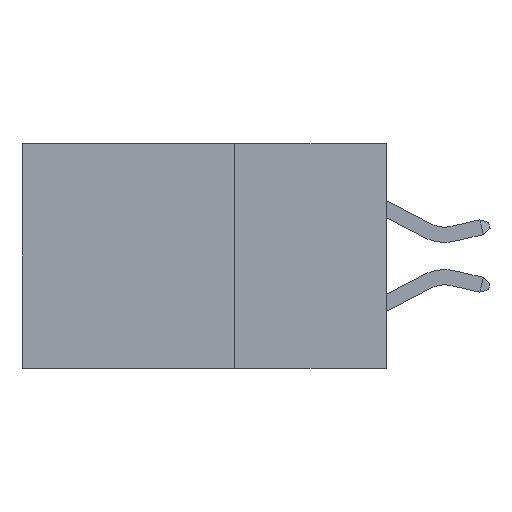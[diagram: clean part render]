
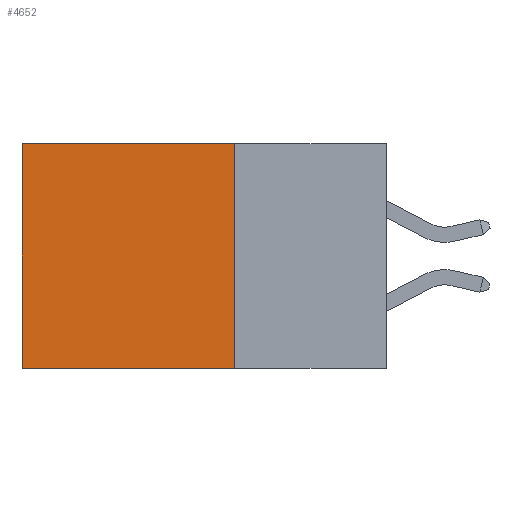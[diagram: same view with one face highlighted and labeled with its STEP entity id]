
A CAD part, left-side view. The second image highlights one B-rep face of the part: STEP entity #4652.
In plain terms, the highlighted planar face has unit normal (-1, 0, 0).
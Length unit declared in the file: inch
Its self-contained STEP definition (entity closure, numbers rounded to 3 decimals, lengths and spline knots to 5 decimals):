
#486 = VERTEX_POINT ( 'NONE', #7137 ) ;
#935 = DIRECTION ( 'NONE',  ( 0., 0., -1. ) ) ;
#1513 = EDGE_LOOP ( 'NONE', ( #7203, #8197, #4393, #14992 ) ) ;
#1805 = VERTEX_POINT ( 'NONE', #5164 ) ;
#1903 = VECTOR ( 'NONE', #11298, 39.37008 ) ;
#1962 = PLANE ( 'NONE',  #3621 ) ;
#1999 = EDGE_CURVE ( 'NONE', #9305, #8215, #7406, .T. ) ;
#2483 = LINE ( 'NONE', #11888, #14597 ) ;
#3140 = CARTESIAN_POINT ( 'NONE',  ( 0.298, 0.6, 0. ) ) ;
#3317 = DIRECTION ( 'NONE',  ( 1., 0., 0. ) ) ;
#3621 = AXIS2_PLACEMENT_3D ( 'NONE', #10617, #3317, #14064 ) ;
#4039 = EDGE_CURVE ( 'NONE', #1805, #486, #2483, .T. ) ;
#4267 = EDGE_CURVE ( 'NONE', #8215, #486, #8233, .T. ) ;
#4270 = VECTOR ( 'NONE', #11641, 39.37008 ) ;
#4393 = ORIENTED_EDGE ( 'NONE', *, *, #6775, .F. ) ;
#4652 = ADVANCED_FACE ( 'NONE', ( #14043 ), #1962, .F. ) ;
#5164 = CARTESIAN_POINT ( 'NONE',  ( 0.298, 0.25, -0.37 ) ) ;
#6775 = EDGE_CURVE ( 'NONE', #9305, #1805, #9060, .T. ) ;
#6930 = CARTESIAN_POINT ( 'NONE',  ( 0.298, 0.25, 0. ) ) ;
#7137 = CARTESIAN_POINT ( 'NONE',  ( 0.298, 0.6, -0.37 ) ) ;
#7202 = CARTESIAN_POINT ( 'NONE',  ( 0.298, 0.25, 0. ) ) ;
#7203 = ORIENTED_EDGE ( 'NONE', *, *, #4267, .T. ) ;
#7313 = CARTESIAN_POINT ( 'NONE',  ( 0.298, 0.25, 0. ) ) ;
#7406 = LINE ( 'NONE', #7202, #4270 ) ;
#8197 = ORIENTED_EDGE ( 'NONE', *, *, #4039, .F. ) ;
#8215 = VERTEX_POINT ( 'NONE', #3140 ) ;
#8233 = LINE ( 'NONE', #11483, #1903 ) ;
#9060 = LINE ( 'NONE', #6930, #14829 ) ;
#9186 = DIRECTION ( 'NONE',  ( 0., 1., 0. ) ) ;
#9305 = VERTEX_POINT ( 'NONE', #7313 ) ;
#10617 = CARTESIAN_POINT ( 'NONE',  ( 0.298, 0.25, 0. ) ) ;
#11298 = DIRECTION ( 'NONE',  ( 0., 0., -1. ) ) ;
#11483 = CARTESIAN_POINT ( 'NONE',  ( 0.298, 0.6, 0. ) ) ;
#11641 = DIRECTION ( 'NONE',  ( 0., 1., 0. ) ) ;
#11888 = CARTESIAN_POINT ( 'NONE',  ( 0.298, 0.25, -0.37 ) ) ;
#14043 = FACE_OUTER_BOUND ( 'NONE', #1513, .T. ) ;
#14064 = DIRECTION ( 'NONE',  ( 0., 0., -1. ) ) ;
#14597 = VECTOR ( 'NONE', #9186, 39.37008 ) ;
#14829 = VECTOR ( 'NONE', #935, 39.37008 ) ;
#14992 = ORIENTED_EDGE ( 'NONE', *, *, #1999, .T. ) ;
